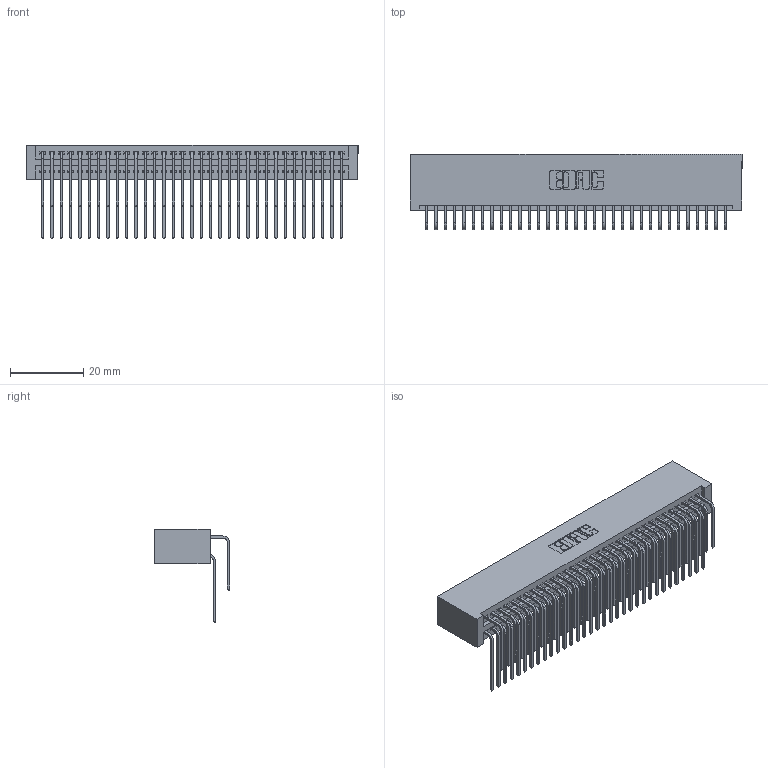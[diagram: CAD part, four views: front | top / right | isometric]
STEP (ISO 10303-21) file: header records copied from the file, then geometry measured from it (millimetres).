
FILE_DESCRIPTION (( 'STEP AP203' ), '1' );
FILE_NAME ('395-066-559-201.STEP', '2018-11-25T06:34:27', ( '' ), ( '' ), 'SwSTEP 2.0', 'SolidWorks 2016', '' );
FILE_SCHEMA (( 'CONFIG_CONTROL_DESIGN' ));
Length unit declared in the file: inch
Products named in the file (4): 345-292-001_559 Tail - 2; 395-066-559-201; 345 Part_No Mounting Lugs; 345-292-001_558 559 Tail - 1
Assembly tree (67 placements, depth 2):
  395-066-559-201
    345 Part_No Mounting Lugs
    345-292-001_558 559 Tail - 1  x33
    345-292-001_559 Tail - 2  x33
Bounding box: 90.42 x 20.56 x 25.53 mm (x, y, z)
Volume: 9697 mm3; surface area: 16253.1 mm2
Topology: 67 solids, 67 shells, 3550 faces, 10547 edges, 6942 vertices
Faces by surface type: plane 2386, cylinder 1164
Entity records: 28479 total; most frequent: CARTESIAN_POINT 4827, ORIENTED_EDGE 4710, DIRECTION 4235, EDGE_CURVE 2355, LINE 2059, VECTOR 2059, VERTEX_POINT 1566, AXIS2_PLACEMENT_3D 1088
